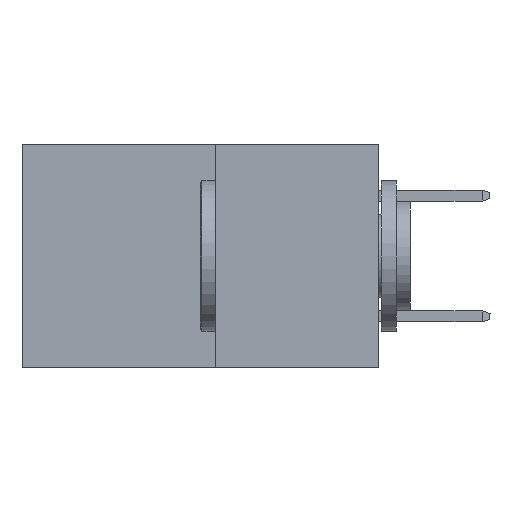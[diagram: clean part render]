
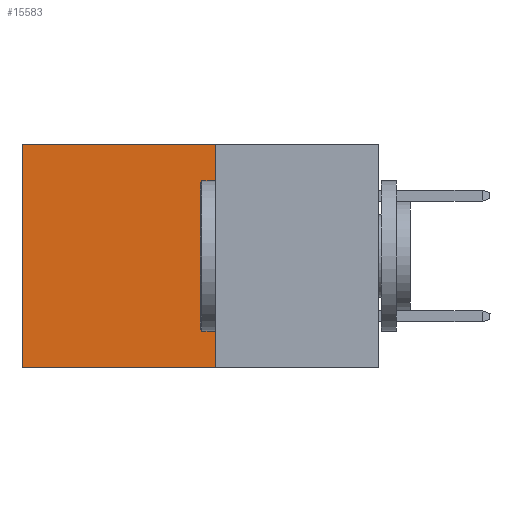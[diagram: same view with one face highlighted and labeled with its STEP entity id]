
A CAD part, left-side view. The second image highlights one B-rep face of the part: STEP entity #15583.
In plain terms, the highlighted planar face has unit normal (-1, 0, 0).
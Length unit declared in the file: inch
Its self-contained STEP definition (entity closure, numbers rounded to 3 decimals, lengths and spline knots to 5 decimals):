
#827 = CARTESIAN_POINT ( 'NONE',  ( 0.277, 0.59, -0.37 ) ) ;
#1263 = CARTESIAN_POINT ( 'NONE',  ( 0.277, 0.27, 0. ) ) ;
#1541 = LINE ( 'NONE', #4803, #20305 ) ;
#2540 = EDGE_CURVE ( 'NONE', #25794, #20846, #25255, .T. ) ;
#3460 = EDGE_CURVE ( 'NONE', #25794, #25458, #19700, .T. ) ;
#3775 = DIRECTION ( 'NONE',  ( 0., 1., 0. ) ) ;
#4797 = DIRECTION ( 'NONE',  ( 0., 1., 0. ) ) ;
#4803 = CARTESIAN_POINT ( 'NONE',  ( 0.277, 0.27, -0.37 ) ) ;
#4924 = PLANE ( 'NONE',  #29477 ) ;
#4935 = ORIENTED_EDGE ( 'NONE', *, *, #5690, .F. ) ;
#5690 = EDGE_CURVE ( 'NONE', #25458, #18665, #1541, .T. ) ;
#6415 = ORIENTED_EDGE ( 'NONE', *, *, #2540, .T. ) ;
#6543 = VECTOR ( 'NONE', #3775, 39.37008 ) ;
#7751 = DIRECTION ( 'NONE',  ( 0., 0., -1. ) ) ;
#8211 = EDGE_LOOP ( 'NONE', ( #9679, #4935, #11165, #6415 ) ) ;
#8779 = CARTESIAN_POINT ( 'NONE',  ( 0.277, 0.27, -0.37 ) ) ;
#9610 = DIRECTION ( 'NONE',  ( 0., 0., -1. ) ) ;
#9679 = ORIENTED_EDGE ( 'NONE', *, *, #18816, .T. ) ;
#11165 = ORIENTED_EDGE ( 'NONE', *, *, #3460, .F. ) ;
#11224 = CARTESIAN_POINT ( 'NONE',  ( 0.277, 0.27, 0. ) ) ;
#11885 = CARTESIAN_POINT ( 'NONE',  ( 0.277, 0.27, -0.37 ) ) ;
#13067 = CARTESIAN_POINT ( 'NONE',  ( 0.277, 0.59, -0.37 ) ) ;
#15583 = ADVANCED_FACE ( 'NONE', ( #22069 ), #4924, .F. ) ;
#18665 = VERTEX_POINT ( 'NONE', #827 ) ;
#18816 = EDGE_CURVE ( 'NONE', #20846, #18665, #27707, .T. ) ;
#19700 = LINE ( 'NONE', #8779, #24467 ) ;
#20305 = VECTOR ( 'NONE', #4797, 39.37008 ) ;
#20846 = VERTEX_POINT ( 'NONE', #28918 ) ;
#21348 = CARTESIAN_POINT ( 'NONE',  ( 0.277, 0.27, -0.37 ) ) ;
#22069 = FACE_OUTER_BOUND ( 'NONE', #8211, .T. ) ;
#23700 = DIRECTION ( 'NONE',  ( 1., 0., 0. ) ) ;
#24467 = VECTOR ( 'NONE', #7751, 39.37008 ) ;
#25255 = LINE ( 'NONE', #11224, #6543 ) ;
#25458 = VERTEX_POINT ( 'NONE', #11885 ) ;
#25794 = VERTEX_POINT ( 'NONE', #1263 ) ;
#26298 = VECTOR ( 'NONE', #27048, 39.37008 ) ;
#27048 = DIRECTION ( 'NONE',  ( 0., 0., -1. ) ) ;
#27707 = LINE ( 'NONE', #13067, #26298 ) ;
#28918 = CARTESIAN_POINT ( 'NONE',  ( 0.277, 0.59, 0. ) ) ;
#29477 = AXIS2_PLACEMENT_3D ( 'NONE', #21348, #23700, #9610 ) ;
